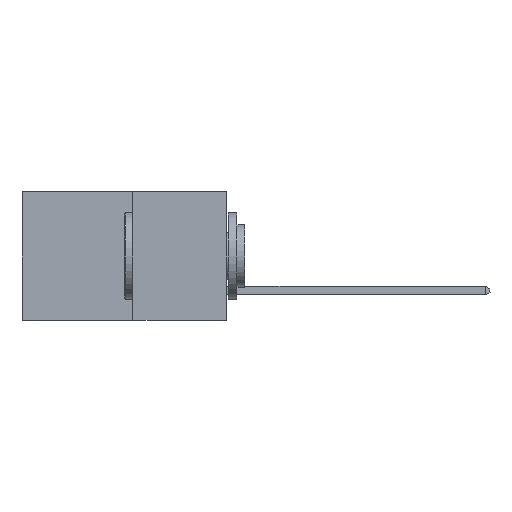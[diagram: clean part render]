
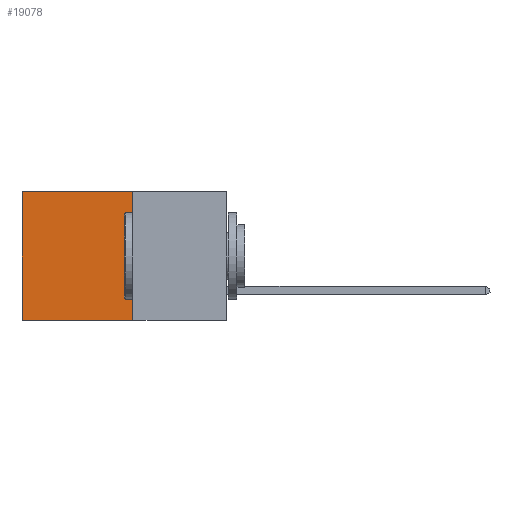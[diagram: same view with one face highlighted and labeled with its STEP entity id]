
A CAD part, left-side view. The second image highlights one B-rep face of the part: STEP entity #19078.
In plain terms, the highlighted planar face has unit normal (-1, 0, 0).
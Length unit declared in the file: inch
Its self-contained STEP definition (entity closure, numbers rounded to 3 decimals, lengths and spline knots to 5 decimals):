
#525 = VERTEX_POINT ( 'NONE', #19407 ) ;
#818 = DIRECTION ( 'NONE',  ( 0., 0., -1. ) ) ;
#2098 = VERTEX_POINT ( 'NONE', #4957 ) ;
#2171 = VECTOR ( 'NONE', #818, 39.37008 ) ;
#2881 = EDGE_CURVE ( 'NONE', #525, #2098, #21089, .T. ) ;
#4062 = VECTOR ( 'NONE', #7823, 39.37008 ) ;
#4474 = ORIENTED_EDGE ( 'NONE', *, *, #24488, .F. ) ;
#4868 = LINE ( 'NONE', #8302, #4062 ) ;
#4957 = CARTESIAN_POINT ( 'NONE',  ( 0.277, 0.59, 0. ) ) ;
#5271 = EDGE_CURVE ( 'NONE', #8357, #12151, #4868, .T. ) ;
#5361 = CARTESIAN_POINT ( 'NONE',  ( 0.277, 0.27, 0. ) ) ;
#5385 = ORIENTED_EDGE ( 'NONE', *, *, #2881, .T. ) ;
#5899 = CARTESIAN_POINT ( 'NONE',  ( 0.277, 0.27, -0.37 ) ) ;
#6273 = DIRECTION ( 'NONE',  ( 0., 1., 0. ) ) ;
#6627 = EDGE_LOOP ( 'NONE', ( #6730, #16822, #4474, #5385 ) ) ;
#6730 = ORIENTED_EDGE ( 'NONE', *, *, #28572, .T. ) ;
#7823 = DIRECTION ( 'NONE',  ( 0., 1., 0. ) ) ;
#8302 = CARTESIAN_POINT ( 'NONE',  ( 0.277, 0.27, -0.37 ) ) ;
#8357 = VERTEX_POINT ( 'NONE', #14752 ) ;
#10144 = AXIS2_PLACEMENT_3D ( 'NONE', #21315, #14029, #26086 ) ;
#10553 = VECTOR ( 'NONE', #17344, 39.37008 ) ;
#12151 = VERTEX_POINT ( 'NONE', #21388 ) ;
#14029 = DIRECTION ( 'NONE',  ( 1., 0., 0. ) ) ;
#14362 = FACE_OUTER_BOUND ( 'NONE', #6627, .T. ) ;
#14752 = CARTESIAN_POINT ( 'NONE',  ( 0.277, 0.27, -0.37 ) ) ;
#16822 = ORIENTED_EDGE ( 'NONE', *, *, #5271, .F. ) ;
#17344 = DIRECTION ( 'NONE',  ( 0., 0., -1. ) ) ;
#17583 = LINE ( 'NONE', #5899, #2171 ) ;
#19078 = ADVANCED_FACE ( 'NONE', ( #14362 ), #23726, .F. ) ;
#19407 = CARTESIAN_POINT ( 'NONE',  ( 0.277, 0.27, 0. ) ) ;
#20321 = VECTOR ( 'NONE', #6273, 39.37008 ) ;
#21089 = LINE ( 'NONE', #5361, #20321 ) ;
#21315 = CARTESIAN_POINT ( 'NONE',  ( 0.277, 0.27, -0.37 ) ) ;
#21388 = CARTESIAN_POINT ( 'NONE',  ( 0.277, 0.59, -0.37 ) ) ;
#23726 = PLANE ( 'NONE',  #10144 ) ;
#24488 = EDGE_CURVE ( 'NONE', #525, #8357, #17583, .T. ) ;
#26086 = DIRECTION ( 'NONE',  ( 0., 0., -1. ) ) ;
#28572 = EDGE_CURVE ( 'NONE', #2098, #12151, #29666, .T. ) ;
#29255 = CARTESIAN_POINT ( 'NONE',  ( 0.277, 0.59, -0.37 ) ) ;
#29666 = LINE ( 'NONE', #29255, #10553 ) ;
